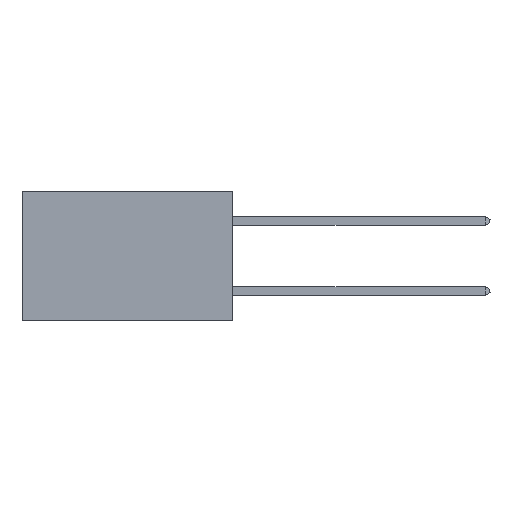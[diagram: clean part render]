
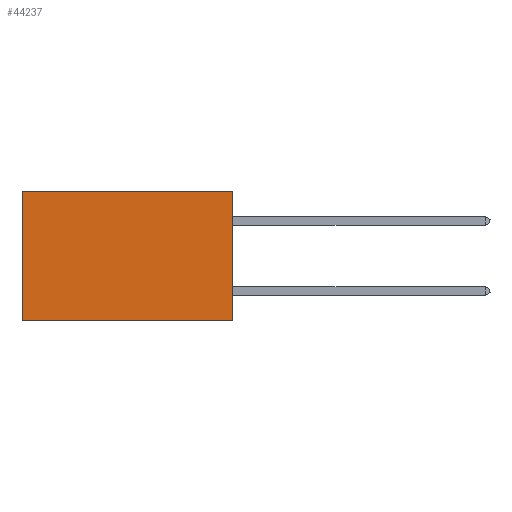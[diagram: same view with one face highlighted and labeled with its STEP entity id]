
A CAD part, left-side view. The second image highlights one B-rep face of the part: STEP entity #44237.
In plain terms, the highlighted planar face has unit normal (-1, 0, 0).
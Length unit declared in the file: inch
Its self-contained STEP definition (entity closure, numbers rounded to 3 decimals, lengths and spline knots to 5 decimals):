
#2544 = PLANE ( 'NONE',  #4527 ) ;
#3011 = DIRECTION ( 'NONE',  ( 0., 0., -1. ) ) ;
#3214 = ORIENTED_EDGE ( 'NONE', *, *, #29700, .F. ) ;
#4527 = AXIS2_PLACEMENT_3D ( 'NONE', #26614, #26764, #3011 ) ;
#6428 = LINE ( 'NONE', #27166, #37797 ) ;
#6684 = VECTOR ( 'NONE', #36861, 39.37008 ) ;
#6835 = VECTOR ( 'NONE', #22479, 39.37008 ) ;
#7810 = CARTESIAN_POINT ( 'NONE',  ( 0.2875, 0.6, -0.37 ) ) ;
#9312 = EDGE_CURVE ( 'NONE', #42104, #32565, #40159, .T. ) ;
#11242 = EDGE_CURVE ( 'NONE', #22102, #37083, #6428, .T. ) ;
#14294 = DIRECTION ( 'NONE',  ( 0., 1., 0. ) ) ;
#14474 = CARTESIAN_POINT ( 'NONE',  ( 0.2875, 0.6, 0. ) ) ;
#16421 = LINE ( 'NONE', #19945, #6684 ) ;
#16508 = ORIENTED_EDGE ( 'NONE', *, *, #11242, .T. ) ;
#17422 = VECTOR ( 'NONE', #14294, 39.37008 ) ;
#17642 = CARTESIAN_POINT ( 'NONE',  ( 0.2875, 0., -0.37 ) ) ;
#19131 = FACE_OUTER_BOUND ( 'NONE', #43880, .T. ) ;
#19945 = CARTESIAN_POINT ( 'NONE',  ( 0.2875, 0.6, 0. ) ) ;
#22102 = VERTEX_POINT ( 'NONE', #38579 ) ;
#22479 = DIRECTION ( 'NONE',  ( 0., 0., -1. ) ) ;
#23809 = DIRECTION ( 'NONE',  ( 0., 1., 0. ) ) ;
#25979 = ORIENTED_EDGE ( 'NONE', *, *, #44398, .T. ) ;
#26614 = CARTESIAN_POINT ( 'NONE',  ( 0.2875, 0., 0. ) ) ;
#26764 = DIRECTION ( 'NONE',  ( 1., 0., 0. ) ) ;
#27166 = CARTESIAN_POINT ( 'NONE',  ( 0.2875, 0., 0. ) ) ;
#29700 = EDGE_CURVE ( 'NONE', #22102, #42104, #42005, .T. ) ;
#31841 = ORIENTED_EDGE ( 'NONE', *, *, #9312, .F. ) ;
#32565 = VERTEX_POINT ( 'NONE', #7810 ) ;
#36861 = DIRECTION ( 'NONE',  ( 0., 0., -1. ) ) ;
#37083 = VERTEX_POINT ( 'NONE', #14474 ) ;
#37797 = VECTOR ( 'NONE', #23809, 39.37008 ) ;
#38579 = CARTESIAN_POINT ( 'NONE',  ( 0.2875, 0., 0. ) ) ;
#39753 = CARTESIAN_POINT ( 'NONE',  ( 0.2875, 0., 0. ) ) ;
#40159 = LINE ( 'NONE', #17642, #17422 ) ;
#40645 = CARTESIAN_POINT ( 'NONE',  ( 0.2875, 0., -0.37 ) ) ;
#42005 = LINE ( 'NONE', #39753, #6835 ) ;
#42104 = VERTEX_POINT ( 'NONE', #40645 ) ;
#43880 = EDGE_LOOP ( 'NONE', ( #25979, #31841, #3214, #16508 ) ) ;
#44237 = ADVANCED_FACE ( 'NONE', ( #19131 ), #2544, .F. ) ;
#44398 = EDGE_CURVE ( 'NONE', #37083, #32565, #16421, .T. ) ;
